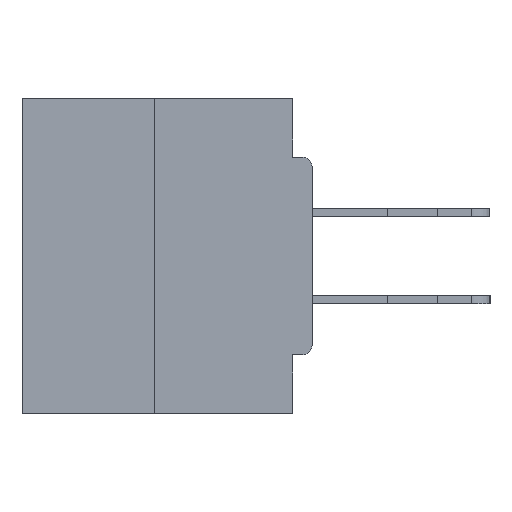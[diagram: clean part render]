
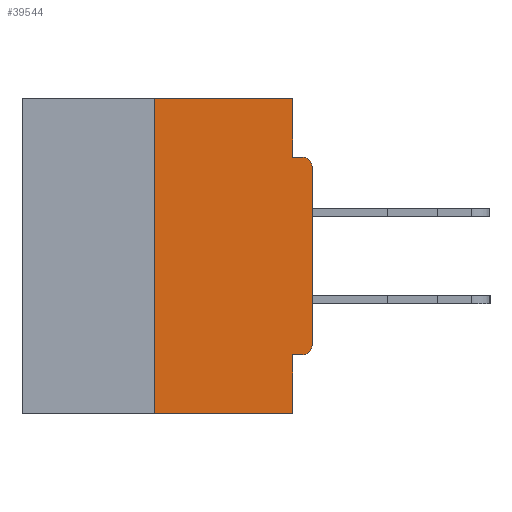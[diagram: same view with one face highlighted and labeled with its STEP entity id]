
A CAD part, left-side view. The second image highlights one B-rep face of the part: STEP entity #39544.
In plain terms, the highlighted planar face has unit normal (-1, 0, 0).
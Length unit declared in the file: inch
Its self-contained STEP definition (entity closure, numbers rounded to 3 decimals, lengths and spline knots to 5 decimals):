
#137 = CARTESIAN_POINT ( 'NONE',  ( 0., 0.031, -0.4065 ) ) ;
#674 = VERTEX_POINT ( 'NONE', #21206 ) ;
#1067 = EDGE_CURVE ( 'NONE', #30192, #4009, #23294, .T. ) ;
#2361 = DIRECTION ( 'NONE',  ( 0., 0., -1. ) ) ;
#2593 = CARTESIAN_POINT ( 'NONE',  ( 0., 0., -0.3915 ) ) ;
#3516 = PLANE ( 'NONE',  #13821 ) ;
#3592 = DIRECTION ( 'NONE',  ( 0., 0., 1. ) ) ;
#3842 = CARTESIAN_POINT ( 'NONE',  ( 0., 0.015, -0.4065 ) ) ;
#4009 = VERTEX_POINT ( 'NONE', #13156 ) ;
#4098 = CARTESIAN_POINT ( 'NONE',  ( 0., 0.015, -0.3915 ) ) ;
#5601 = VECTOR ( 'NONE', #39995, 39.37008 ) ;
#6205 = VECTOR ( 'NONE', #32478, 39.37008 ) ;
#6284 = CARTESIAN_POINT ( 'NONE',  ( 0., 0., -0.1085 ) ) ;
#6839 = CIRCLE ( 'NONE', #28376, 0.015 ) ;
#7084 = ORIENTED_EDGE ( 'NONE', *, *, #29595, .F. ) ;
#7488 = LINE ( 'NONE', #12983, #16351 ) ;
#7703 = FACE_OUTER_BOUND ( 'NONE', #10489, .T. ) ;
#7708 = CARTESIAN_POINT ( 'NONE',  ( 0., 0.015, -0.0935 ) ) ;
#8024 = CARTESIAN_POINT ( 'NONE',  ( 0., 0.46, 0. ) ) ;
#8301 = ORIENTED_EDGE ( 'NONE', *, *, #9022, .T. ) ;
#9022 = EDGE_CURVE ( 'NONE', #31548, #14645, #15741, .T. ) ;
#10489 = EDGE_LOOP ( 'NONE', ( #7084, #37940, #20212, #16328, #26128, #35489, #8301, #24958, #26017, #27236 ) ) ;
#10637 = EDGE_CURVE ( 'NONE', #14645, #25817, #21940, .T. ) ;
#12844 = DIRECTION ( 'NONE',  ( 1., 0., 0. ) ) ;
#12983 = CARTESIAN_POINT ( 'NONE',  ( 0., 0., -0.4065 ) ) ;
#13058 = CARTESIAN_POINT ( 'NONE',  ( 0., 0., 0. ) ) ;
#13156 = CARTESIAN_POINT ( 'NONE',  ( 0., 0.031, -0.0935 ) ) ;
#13821 = AXIS2_PLACEMENT_3D ( 'NONE', #15595, #12844, #31644 ) ;
#14098 = CARTESIAN_POINT ( 'NONE',  ( 0., 0.25, 0. ) ) ;
#14225 = VERTEX_POINT ( 'NONE', #3842 ) ;
#14645 = VERTEX_POINT ( 'NONE', #6284 ) ;
#15043 = VECTOR ( 'NONE', #39239, 39.37008 ) ;
#15418 = LINE ( 'NONE', #33751, #23292 ) ;
#15595 = CARTESIAN_POINT ( 'NONE',  ( 0., 0.46, 0. ) ) ;
#15741 = LINE ( 'NONE', #13058, #31439 ) ;
#16328 = ORIENTED_EDGE ( 'NONE', *, *, #16935, .F. ) ;
#16351 = VECTOR ( 'NONE', #23345, 39.37008 ) ;
#16935 = EDGE_CURVE ( 'NONE', #39015, #674, #15418, .T. ) ;
#17623 = VERTEX_POINT ( 'NONE', #31519 ) ;
#18005 = EDGE_CURVE ( 'NONE', #17623, #22051, #25337, .T. ) ;
#19316 = CARTESIAN_POINT ( 'NONE',  ( 0., 0.46, -0.5 ) ) ;
#19927 = LINE ( 'NONE', #35509, #6205 ) ;
#20212 = ORIENTED_EDGE ( 'NONE', *, *, #26804, .T. ) ;
#20305 = EDGE_CURVE ( 'NONE', #14225, #39015, #7488, .T. ) ;
#21143 = DIRECTION ( 'NONE',  ( -1., 0., 0. ) ) ;
#21151 = VECTOR ( 'NONE', #31708, 39.37008 ) ;
#21206 = CARTESIAN_POINT ( 'NONE',  ( 0., 0.031, -0.5 ) ) ;
#21631 = LINE ( 'NONE', #19316, #21151 ) ;
#21940 = CIRCLE ( 'NONE', #37735, 0.015 ) ;
#22051 = VERTEX_POINT ( 'NONE', #27375 ) ;
#23292 = VECTOR ( 'NONE', #27841, 39.37008 ) ;
#23294 = LINE ( 'NONE', #23383, #5601 ) ;
#23345 = DIRECTION ( 'NONE',  ( 0., 1., 0. ) ) ;
#23383 = CARTESIAN_POINT ( 'NONE',  ( 0., 0.031, 0. ) ) ;
#24332 = DIRECTION ( 'NONE',  ( 0., 0., -1. ) ) ;
#24958 = ORIENTED_EDGE ( 'NONE', *, *, #10637, .T. ) ;
#25337 = LINE ( 'NONE', #14098, #15043 ) ;
#25817 = VERTEX_POINT ( 'NONE', #7708 ) ;
#26017 = ORIENTED_EDGE ( 'NONE', *, *, #39651, .F. ) ;
#26128 = ORIENTED_EDGE ( 'NONE', *, *, #20305, .F. ) ;
#26804 = EDGE_CURVE ( 'NONE', #17623, #674, #21631, .T. ) ;
#27236 = ORIENTED_EDGE ( 'NONE', *, *, #1067, .F. ) ;
#27375 = CARTESIAN_POINT ( 'NONE',  ( 0., 0.25, 0. ) ) ;
#27841 = DIRECTION ( 'NONE',  ( 0., 0., -1. ) ) ;
#28376 = AXIS2_PLACEMENT_3D ( 'NONE', #4098, #21143, #2361 ) ;
#29595 = EDGE_CURVE ( 'NONE', #22051, #30192, #32742, .T. ) ;
#30192 = VERTEX_POINT ( 'NONE', #37649 ) ;
#31042 = EDGE_CURVE ( 'NONE', #14225, #31548, #6839, .T. ) ;
#31439 = VECTOR ( 'NONE', #3592, 39.37008 ) ;
#31519 = CARTESIAN_POINT ( 'NONE',  ( 0., 0.25, -0.5 ) ) ;
#31548 = VERTEX_POINT ( 'NONE', #2593 ) ;
#31644 = DIRECTION ( 'NONE',  ( 0., 0., -1. ) ) ;
#31708 = DIRECTION ( 'NONE',  ( 0., -1., 0. ) ) ;
#32478 = DIRECTION ( 'NONE',  ( 0., -1., 0. ) ) ;
#32742 = LINE ( 'NONE', #8024, #34191 ) ;
#33751 = CARTESIAN_POINT ( 'NONE',  ( 0., 0.031, -0.5 ) ) ;
#34191 = VECTOR ( 'NONE', #36741, 39.37008 ) ;
#34242 = CARTESIAN_POINT ( 'NONE',  ( 0., 0.015, -0.1085 ) ) ;
#35489 = ORIENTED_EDGE ( 'NONE', *, *, #31042, .T. ) ;
#35509 = CARTESIAN_POINT ( 'NONE',  ( 0., 0., -0.0935 ) ) ;
#36741 = DIRECTION ( 'NONE',  ( 0., -1., 0. ) ) ;
#37001 = DIRECTION ( 'NONE',  ( -1., 0., 0. ) ) ;
#37649 = CARTESIAN_POINT ( 'NONE',  ( 0., 0.031, 0. ) ) ;
#37735 = AXIS2_PLACEMENT_3D ( 'NONE', #34242, #37001, #24332 ) ;
#37940 = ORIENTED_EDGE ( 'NONE', *, *, #18005, .F. ) ;
#39015 = VERTEX_POINT ( 'NONE', #137 ) ;
#39239 = DIRECTION ( 'NONE',  ( 0., 0., 1. ) ) ;
#39544 = ADVANCED_FACE ( 'NONE', ( #7703 ), #3516, .F. ) ;
#39651 = EDGE_CURVE ( 'NONE', #4009, #25817, #19927, .T. ) ;
#39995 = DIRECTION ( 'NONE',  ( 0., 0., -1. ) ) ;
